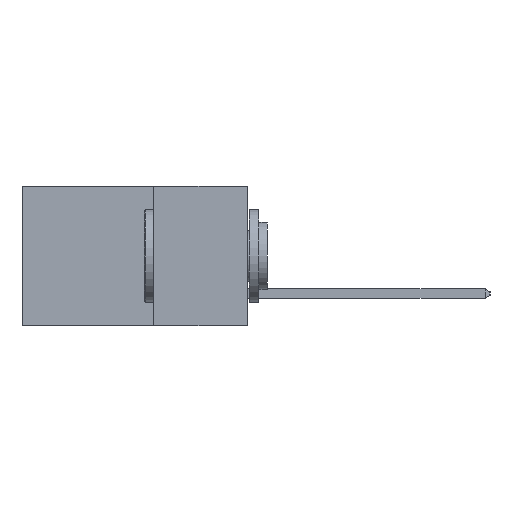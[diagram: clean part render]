
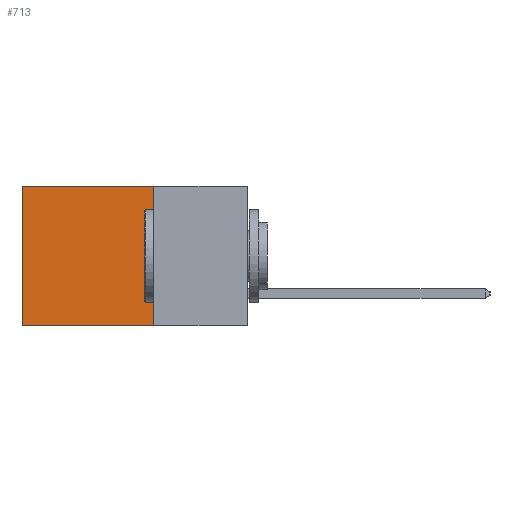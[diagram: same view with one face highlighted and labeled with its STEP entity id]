
A CAD part, left-side view. The second image highlights one B-rep face of the part: STEP entity #713.
In plain terms, the highlighted planar face has unit normal (-1, 0, 0).
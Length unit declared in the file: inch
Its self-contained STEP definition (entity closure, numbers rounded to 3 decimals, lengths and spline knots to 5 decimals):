
#713 = ADVANCED_FACE ( 'NONE', ( #6133 ), #14836, .F. ) ;
#2195 = CARTESIAN_POINT ( 'NONE',  ( 0.298, 0.25, 0. ) ) ;
#2210 = CARTESIAN_POINT ( 'NONE',  ( 0.298, 0.6, 0. ) ) ;
#4332 = DIRECTION ( 'NONE',  ( 1., 0., 0. ) ) ;
#4642 = CARTESIAN_POINT ( 'NONE',  ( 0.298, 0.25, 0. ) ) ;
#4717 = VECTOR ( 'NONE', #10007, 39.37008 ) ;
#4781 = LINE ( 'NONE', #17795, #5248 ) ;
#5046 = CARTESIAN_POINT ( 'NONE',  ( 0.298, 0.25, -0.37 ) ) ;
#5248 = VECTOR ( 'NONE', #6965, 39.37008 ) ;
#5252 = ORIENTED_EDGE ( 'NONE', *, *, #9805, .T. ) ;
#5895 = EDGE_CURVE ( 'NONE', #9692, #11219, #6498, .T. ) ;
#6025 = VECTOR ( 'NONE', #12302, 39.37008 ) ;
#6133 = FACE_OUTER_BOUND ( 'NONE', #12718, .T. ) ;
#6498 = LINE ( 'NONE', #4642, #6025 ) ;
#6965 = DIRECTION ( 'NONE',  ( 0., 0., -1. ) ) ;
#7149 = CARTESIAN_POINT ( 'NONE',  ( 0.298, 0.25, -0.37 ) ) ;
#7545 = VECTOR ( 'NONE', #14335, 39.37008 ) ;
#8425 = CARTESIAN_POINT ( 'NONE',  ( 0.298, 0.6, 0. ) ) ;
#8452 = ORIENTED_EDGE ( 'NONE', *, *, #5895, .T. ) ;
#8485 = EDGE_CURVE ( 'NONE', #9692, #17849, #4781, .T. ) ;
#8664 = ORIENTED_EDGE ( 'NONE', *, *, #15037, .F. ) ;
#9692 = VERTEX_POINT ( 'NONE', #2195 ) ;
#9805 = EDGE_CURVE ( 'NONE', #11219, #11082, #12971, .T. ) ;
#10007 = DIRECTION ( 'NONE',  ( 0., 0., -1. ) ) ;
#11082 = VERTEX_POINT ( 'NONE', #15707 ) ;
#11219 = VERTEX_POINT ( 'NONE', #2210 ) ;
#12302 = DIRECTION ( 'NONE',  ( 0., 1., 0. ) ) ;
#12579 = ORIENTED_EDGE ( 'NONE', *, *, #8485, .F. ) ;
#12718 = EDGE_LOOP ( 'NONE', ( #5252, #8664, #12579, #8452 ) ) ;
#12971 = LINE ( 'NONE', #8425, #4717 ) ;
#13919 = AXIS2_PLACEMENT_3D ( 'NONE', #15256, #4332, #17842 ) ;
#14335 = DIRECTION ( 'NONE',  ( 0., 1., 0. ) ) ;
#14836 = PLANE ( 'NONE',  #13919 ) ;
#15037 = EDGE_CURVE ( 'NONE', #17849, #11082, #19306, .T. ) ;
#15256 = CARTESIAN_POINT ( 'NONE',  ( 0.298, 0.25, 0. ) ) ;
#15707 = CARTESIAN_POINT ( 'NONE',  ( 0.298, 0.6, -0.37 ) ) ;
#17795 = CARTESIAN_POINT ( 'NONE',  ( 0.298, 0.25, 0. ) ) ;
#17842 = DIRECTION ( 'NONE',  ( 0., 0., -1. ) ) ;
#17849 = VERTEX_POINT ( 'NONE', #7149 ) ;
#19306 = LINE ( 'NONE', #5046, #7545 ) ;
